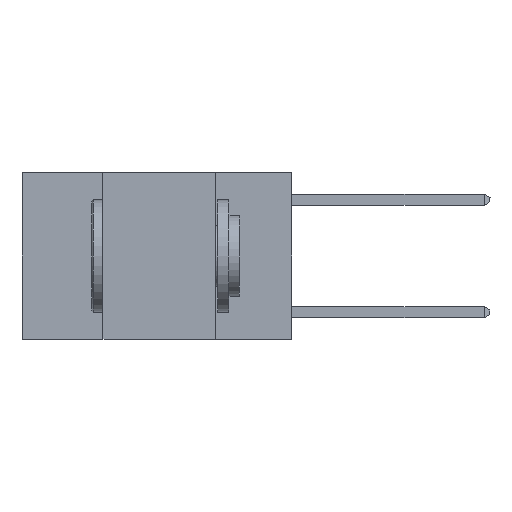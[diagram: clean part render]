
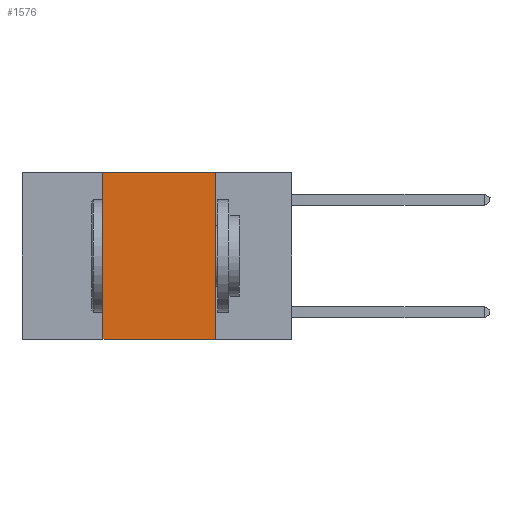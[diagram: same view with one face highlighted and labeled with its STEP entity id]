
A CAD part, left-side view. The second image highlights one B-rep face of the part: STEP entity #1576.
In plain terms, the highlighted planar face has unit normal (-1, 0, 0).
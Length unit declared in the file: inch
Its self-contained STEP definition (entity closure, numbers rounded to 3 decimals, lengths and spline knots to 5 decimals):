
#111 = EDGE_LOOP ( 'NONE', ( #16411, #16428, #16815, #16834 ) ) ;
#1181 = CARTESIAN_POINT ( 'NONE',  ( 0., 0.42, 0. ) ) ;
#1576 = ADVANCED_FACE ( 'NONE', ( #2002 ), #3348, .F. ) ;
#2002 = FACE_OUTER_BOUND ( 'NONE', #111, .T. ) ;
#2391 = EDGE_CURVE ( 'NONE', #16768, #17064, #7701, .T. ) ;
#2486 = CARTESIAN_POINT ( 'NONE',  ( 0., 0.17, -0.37 ) ) ;
#2749 = LINE ( 'NONE', #3903, #13038 ) ;
#2996 = DIRECTION ( 'NONE',  ( 0., 0., -1. ) ) ;
#3272 = DIRECTION ( 'NONE',  ( 0., -1., 0. ) ) ;
#3348 = PLANE ( 'NONE',  #7249 ) ;
#3503 = DIRECTION ( 'NONE',  ( 1., 0., 0. ) ) ;
#3739 = VECTOR ( 'NONE', #7113, 39.37008 ) ;
#3903 = CARTESIAN_POINT ( 'NONE',  ( 0., 0.42, 0. ) ) ;
#4027 = CARTESIAN_POINT ( 'NONE',  ( 0., 0.6, 0. ) ) ;
#5266 = DIRECTION ( 'NONE',  ( 0., 0., 1. ) ) ;
#5950 = CARTESIAN_POINT ( 'NONE',  ( 0., 0.6, -0.37 ) ) ;
#6090 = CARTESIAN_POINT ( 'NONE',  ( 0., 0.17, 0. ) ) ;
#7113 = DIRECTION ( 'NONE',  ( 0., 0., -1. ) ) ;
#7249 = AXIS2_PLACEMENT_3D ( 'NONE', #4027, #3503, #2996 ) ;
#7479 = EDGE_CURVE ( 'NONE', #7802, #17064, #16671, .T. ) ;
#7701 = LINE ( 'NONE', #9743, #3739 ) ;
#7802 = VERTEX_POINT ( 'NONE', #13094 ) ;
#9743 = CARTESIAN_POINT ( 'NONE',  ( 0., 0.17, 0. ) ) ;
#10933 = VECTOR ( 'NONE', #14775, 39.37008 ) ;
#11986 = CARTESIAN_POINT ( 'NONE',  ( 0., 0.6, 0. ) ) ;
#12304 = EDGE_CURVE ( 'NONE', #17151, #16768, #14560, .T. ) ;
#13038 = VECTOR ( 'NONE', #5266, 39.37008 ) ;
#13094 = CARTESIAN_POINT ( 'NONE',  ( 0., 0.42, -0.37 ) ) ;
#13194 = VECTOR ( 'NONE', #3272, 39.37008 ) ;
#13674 = EDGE_CURVE ( 'NONE', #7802, #17151, #2749, .T. ) ;
#14560 = LINE ( 'NONE', #11986, #10933 ) ;
#14775 = DIRECTION ( 'NONE',  ( 0., -1., 0. ) ) ;
#16411 = ORIENTED_EDGE ( 'NONE', *, *, #2391, .F. ) ;
#16428 = ORIENTED_EDGE ( 'NONE', *, *, #12304, .F. ) ;
#16671 = LINE ( 'NONE', #5950, #13194 ) ;
#16768 = VERTEX_POINT ( 'NONE', #6090 ) ;
#16815 = ORIENTED_EDGE ( 'NONE', *, *, #13674, .F. ) ;
#16834 = ORIENTED_EDGE ( 'NONE', *, *, #7479, .T. ) ;
#17064 = VERTEX_POINT ( 'NONE', #2486 ) ;
#17151 = VERTEX_POINT ( 'NONE', #1181 ) ;
